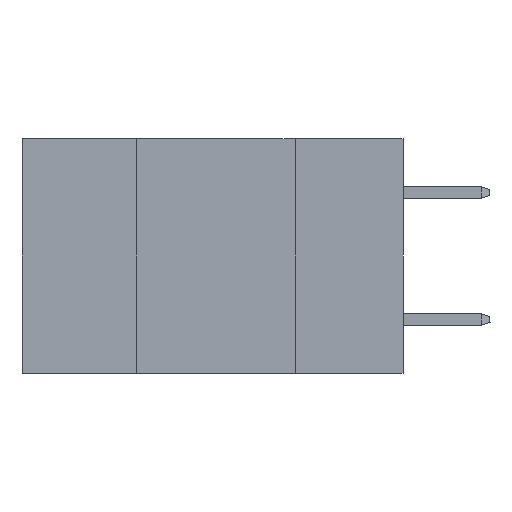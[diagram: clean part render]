
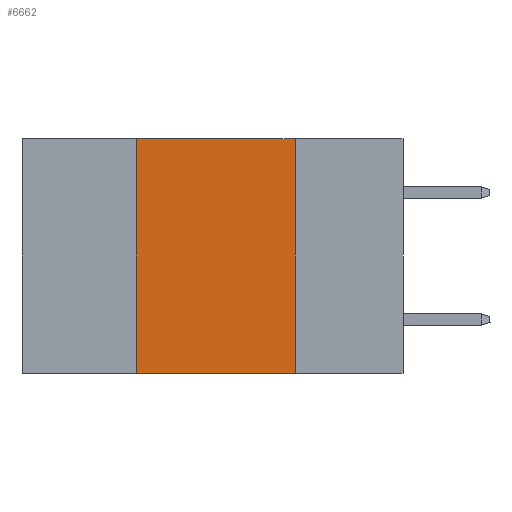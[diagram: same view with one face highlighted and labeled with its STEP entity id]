
A CAD part, left-side view. The second image highlights one B-rep face of the part: STEP entity #6662.
In plain terms, the highlighted planar face has unit normal (-1, 0, 0).
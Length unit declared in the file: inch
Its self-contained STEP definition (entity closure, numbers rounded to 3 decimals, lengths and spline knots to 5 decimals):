
#807 = EDGE_CURVE ( 'NONE', #9075, #11410, #7105, .T. ) ;
#1630 = ORIENTED_EDGE ( 'NONE', *, *, #11809, .F. ) ;
#2619 = EDGE_LOOP ( 'NONE', ( #7712, #1630, #4059, #14006 ) ) ;
#4059 = ORIENTED_EDGE ( 'NONE', *, *, #807, .F. ) ;
#4138 = DIRECTION ( 'NONE',  ( 0., -1., 0. ) ) ;
#4289 = VECTOR ( 'NONE', #4138, 39.37008 ) ;
#5248 = CARTESIAN_POINT ( 'NONE',  ( 0., 0.6, 0. ) ) ;
#5582 = EDGE_CURVE ( 'NONE', #14680, #20512, #16860, .T. ) ;
#5829 = CARTESIAN_POINT ( 'NONE',  ( 0., 0.17, 0. ) ) ;
#6000 = LINE ( 'NONE', #22515, #4289 ) ;
#6428 = VECTOR ( 'NONE', #12884, 39.37008 ) ;
#6662 = ADVANCED_FACE ( 'NONE', ( #20067 ), #10626, .F. ) ;
#6848 = AXIS2_PLACEMENT_3D ( 'NONE', #5248, #23740, #12665 ) ;
#6859 = CARTESIAN_POINT ( 'NONE',  ( 0., 0.17, -0.37 ) ) ;
#7105 = LINE ( 'NONE', #9291, #14752 ) ;
#7712 = ORIENTED_EDGE ( 'NONE', *, *, #5582, .F. ) ;
#9075 = VERTEX_POINT ( 'NONE', #20694 ) ;
#9291 = CARTESIAN_POINT ( 'NONE',  ( 0., 0.42, 0. ) ) ;
#9728 = LINE ( 'NONE', #15259, #17420 ) ;
#10626 = PLANE ( 'NONE',  #6848 ) ;
#11410 = VERTEX_POINT ( 'NONE', #12630 ) ;
#11809 = EDGE_CURVE ( 'NONE', #11410, #14680, #9728, .T. ) ;
#12630 = CARTESIAN_POINT ( 'NONE',  ( 0., 0.42, 0. ) ) ;
#12665 = DIRECTION ( 'NONE',  ( 0., 0., -1. ) ) ;
#12884 = DIRECTION ( 'NONE',  ( 0., 0., -1. ) ) ;
#13030 = DIRECTION ( 'NONE',  ( 0., 0., 1. ) ) ;
#14006 = ORIENTED_EDGE ( 'NONE', *, *, #23964, .T. ) ;
#14680 = VERTEX_POINT ( 'NONE', #20482 ) ;
#14752 = VECTOR ( 'NONE', #13030, 39.37008 ) ;
#15259 = CARTESIAN_POINT ( 'NONE',  ( 0., 0.6, 0. ) ) ;
#16860 = LINE ( 'NONE', #5829, #6428 ) ;
#17090 = DIRECTION ( 'NONE',  ( 0., -1., 0. ) ) ;
#17420 = VECTOR ( 'NONE', #17090, 39.37008 ) ;
#20067 = FACE_OUTER_BOUND ( 'NONE', #2619, .T. ) ;
#20482 = CARTESIAN_POINT ( 'NONE',  ( 0., 0.17, 0. ) ) ;
#20512 = VERTEX_POINT ( 'NONE', #6859 ) ;
#20694 = CARTESIAN_POINT ( 'NONE',  ( 0., 0.42, -0.37 ) ) ;
#22515 = CARTESIAN_POINT ( 'NONE',  ( 0., 0.6, -0.37 ) ) ;
#23740 = DIRECTION ( 'NONE',  ( 1., 0., 0. ) ) ;
#23964 = EDGE_CURVE ( 'NONE', #9075, #20512, #6000, .T. ) ;
